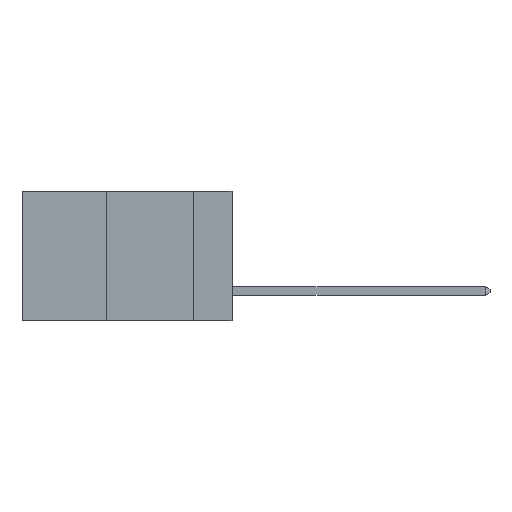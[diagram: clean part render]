
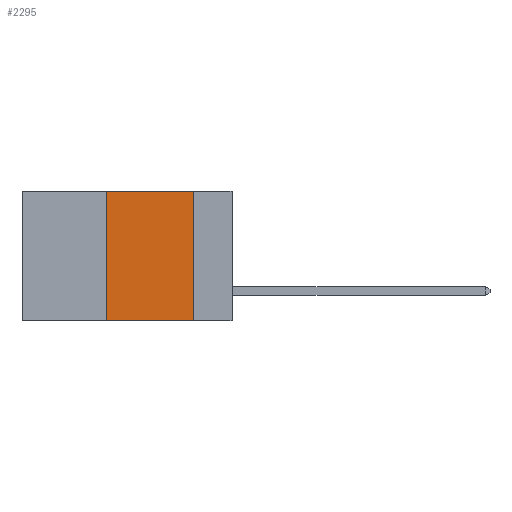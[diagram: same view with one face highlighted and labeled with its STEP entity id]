
A CAD part, left-side view. The second image highlights one B-rep face of the part: STEP entity #2295.
In plain terms, the highlighted planar face has unit normal (-1, 0, 0).
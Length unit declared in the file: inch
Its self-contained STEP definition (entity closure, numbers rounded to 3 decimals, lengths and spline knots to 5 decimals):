
#854 = VECTOR ( 'NONE', #17549, 39.37008 ) ;
#1389 = CARTESIAN_POINT ( 'NONE',  ( 0., 0.6, 0. ) ) ;
#1757 = FACE_OUTER_BOUND ( 'NONE', #3436, .T. ) ;
#2295 = ADVANCED_FACE ( 'NONE', ( #1757 ), #16397, .F. ) ;
#2923 = CARTESIAN_POINT ( 'NONE',  ( 0., 0.6, -0.37 ) ) ;
#3436 = EDGE_LOOP ( 'NONE', ( #10716, #15515, #6364, #20853 ) ) ;
#4094 = VERTEX_POINT ( 'NONE', #9919 ) ;
#4388 = DIRECTION ( 'NONE',  ( 0., 0., 1. ) ) ;
#5774 = LINE ( 'NONE', #2923, #854 ) ;
#6364 = ORIENTED_EDGE ( 'NONE', *, *, #10621, .F. ) ;
#7383 = LINE ( 'NONE', #15668, #17594 ) ;
#7407 = VERTEX_POINT ( 'NONE', #15381 ) ;
#7680 = LINE ( 'NONE', #15393, #16762 ) ;
#8142 = EDGE_CURVE ( 'NONE', #4094, #7407, #7383, .T. ) ;
#8447 = AXIS2_PLACEMENT_3D ( 'NONE', #10968, #20021, #9208 ) ;
#8874 = DIRECTION ( 'NONE',  ( 0., -1., 0. ) ) ;
#9208 = DIRECTION ( 'NONE',  ( 0., 0., -1. ) ) ;
#9919 = CARTESIAN_POINT ( 'NONE',  ( 0., 0.11, 0. ) ) ;
#10621 = EDGE_CURVE ( 'NONE', #23165, #16425, #7680, .T. ) ;
#10716 = ORIENTED_EDGE ( 'NONE', *, *, #8142, .F. ) ;
#10968 = CARTESIAN_POINT ( 'NONE',  ( 0., 0.6, 0. ) ) ;
#12127 = VECTOR ( 'NONE', #8874, 39.37008 ) ;
#12744 = CARTESIAN_POINT ( 'NONE',  ( 0., 0.36, 0. ) ) ;
#15381 = CARTESIAN_POINT ( 'NONE',  ( 0., 0.11, -0.37 ) ) ;
#15393 = CARTESIAN_POINT ( 'NONE',  ( 0., 0.36, 0. ) ) ;
#15515 = ORIENTED_EDGE ( 'NONE', *, *, #20650, .F. ) ;
#15668 = CARTESIAN_POINT ( 'NONE',  ( 0., 0.11, 0. ) ) ;
#16363 = CARTESIAN_POINT ( 'NONE',  ( 0., 0.36, -0.37 ) ) ;
#16397 = PLANE ( 'NONE',  #8447 ) ;
#16425 = VERTEX_POINT ( 'NONE', #12744 ) ;
#16762 = VECTOR ( 'NONE', #4388, 39.37008 ) ;
#16898 = LINE ( 'NONE', #1389, #12127 ) ;
#17549 = DIRECTION ( 'NONE',  ( 0., -1., 0. ) ) ;
#17594 = VECTOR ( 'NONE', #21088, 39.37008 ) ;
#18704 = EDGE_CURVE ( 'NONE', #23165, #7407, #5774, .T. ) ;
#20021 = DIRECTION ( 'NONE',  ( 1., 0., 0. ) ) ;
#20650 = EDGE_CURVE ( 'NONE', #16425, #4094, #16898, .T. ) ;
#20853 = ORIENTED_EDGE ( 'NONE', *, *, #18704, .T. ) ;
#21088 = DIRECTION ( 'NONE',  ( 0., 0., -1. ) ) ;
#23165 = VERTEX_POINT ( 'NONE', #16363 ) ;
